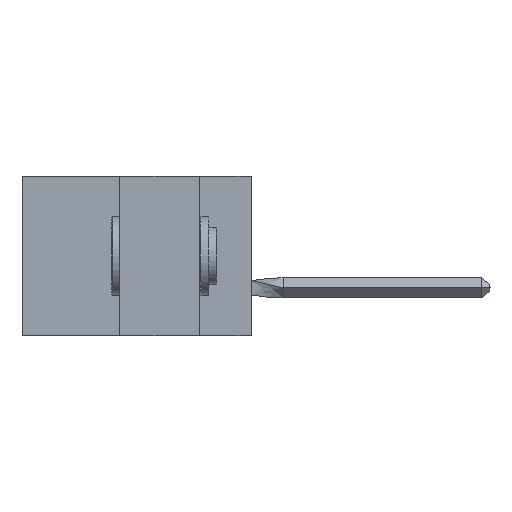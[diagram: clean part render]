
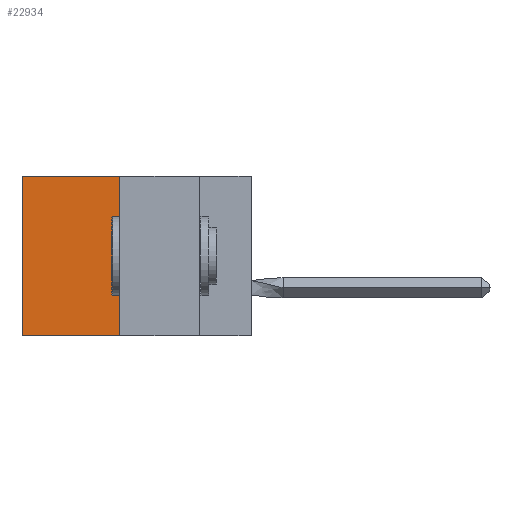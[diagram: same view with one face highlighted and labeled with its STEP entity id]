
A CAD part, left-side view. The second image highlights one B-rep face of the part: STEP entity #22934.
In plain terms, the highlighted planar face has unit normal (-1, 0, 0).
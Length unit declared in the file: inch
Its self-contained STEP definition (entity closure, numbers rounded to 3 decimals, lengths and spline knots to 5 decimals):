
#145 = VECTOR ( 'NONE', #26556, 39.37008 ) ;
#148 = LINE ( 'NONE', #13762, #23646 ) ;
#1005 = DIRECTION ( 'NONE',  ( 0., 1., 0. ) ) ;
#1386 = VERTEX_POINT ( 'NONE', #7755 ) ;
#2000 = EDGE_CURVE ( 'NONE', #1386, #4147, #13492, .T. ) ;
#2154 = DIRECTION ( 'NONE',  ( 0., 0., -1. ) ) ;
#4147 = VERTEX_POINT ( 'NONE', #26936 ) ;
#4636 = ORIENTED_EDGE ( 'NONE', *, *, #8171, .F. ) ;
#6282 = VERTEX_POINT ( 'NONE', #16096 ) ;
#7604 = VECTOR ( 'NONE', #1005, 39.37008 ) ;
#7755 = CARTESIAN_POINT ( 'NONE',  ( 0.305, 0.413, -0.5 ) ) ;
#7817 = AXIS2_PLACEMENT_3D ( 'NONE', #23649, #11891, #2154 ) ;
#8171 = EDGE_CURVE ( 'NONE', #6282, #1386, #28534, .T. ) ;
#8935 = CARTESIAN_POINT ( 'NONE',  ( 0.305, 0.72, 0. ) ) ;
#9706 = EDGE_LOOP ( 'NONE', ( #18840, #19903, #4636, #28724 ) ) ;
#11891 = DIRECTION ( 'NONE',  ( 1., 0., 0. ) ) ;
#13492 = LINE ( 'NONE', #30764, #26927 ) ;
#13762 = CARTESIAN_POINT ( 'NONE',  ( 0.305, 0.72, -0.5 ) ) ;
#14454 = DIRECTION ( 'NONE',  ( 0., 1., 0. ) ) ;
#16096 = CARTESIAN_POINT ( 'NONE',  ( 0.305, 0.413, 0. ) ) ;
#17275 = CARTESIAN_POINT ( 'NONE',  ( 0.305, 0.413, -0.5 ) ) ;
#18418 = LINE ( 'NONE', #24791, #7604 ) ;
#18840 = ORIENTED_EDGE ( 'NONE', *, *, #22890, .T. ) ;
#19238 = EDGE_CURVE ( 'NONE', #6282, #20869, #18418, .T. ) ;
#19903 = ORIENTED_EDGE ( 'NONE', *, *, #2000, .F. ) ;
#20869 = VERTEX_POINT ( 'NONE', #8935 ) ;
#21139 = PLANE ( 'NONE',  #7817 ) ;
#22890 = EDGE_CURVE ( 'NONE', #20869, #4147, #148, .T. ) ;
#22934 = ADVANCED_FACE ( 'NONE', ( #28906 ), #21139, .F. ) ;
#23646 = VECTOR ( 'NONE', #30075, 39.37008 ) ;
#23649 = CARTESIAN_POINT ( 'NONE',  ( 0.305, 0.413, -0.5 ) ) ;
#24791 = CARTESIAN_POINT ( 'NONE',  ( 0.305, 0.413, 0. ) ) ;
#26556 = DIRECTION ( 'NONE',  ( 0., 0., -1. ) ) ;
#26927 = VECTOR ( 'NONE', #14454, 39.37008 ) ;
#26936 = CARTESIAN_POINT ( 'NONE',  ( 0.305, 0.72, -0.5 ) ) ;
#28534 = LINE ( 'NONE', #17275, #145 ) ;
#28724 = ORIENTED_EDGE ( 'NONE', *, *, #19238, .T. ) ;
#28906 = FACE_OUTER_BOUND ( 'NONE', #9706, .T. ) ;
#30075 = DIRECTION ( 'NONE',  ( 0., 0., -1. ) ) ;
#30764 = CARTESIAN_POINT ( 'NONE',  ( 0.305, 0.413, -0.5 ) ) ;
